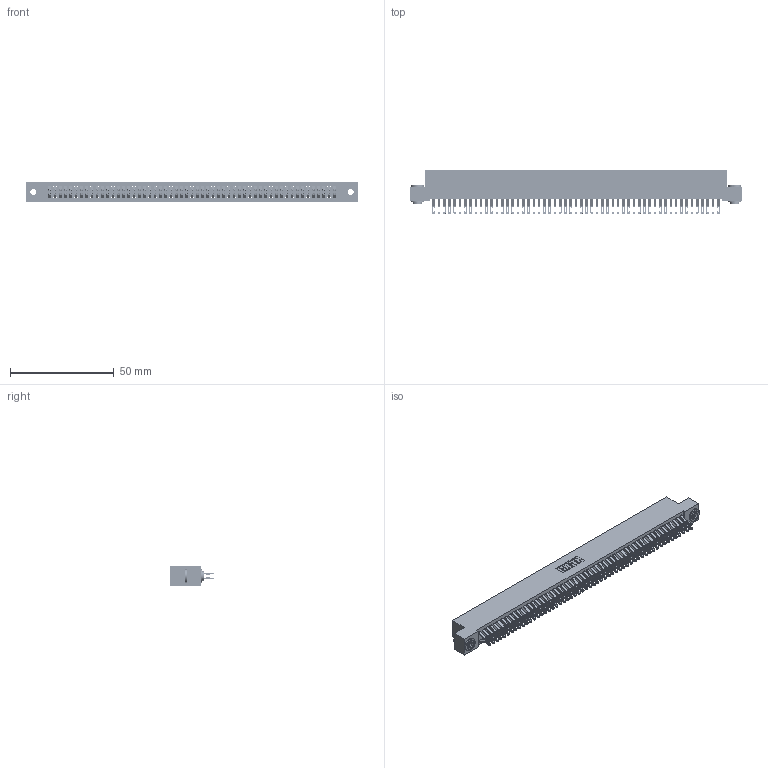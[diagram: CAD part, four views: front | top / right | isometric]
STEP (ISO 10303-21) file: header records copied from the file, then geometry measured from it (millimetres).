
FILE_DESCRIPTION (( 'STEP AP203' ), '1' );
FILE_NAME ('342-110-555-203.STEP', '2018-08-14T11:41:17', ( '' ), ( '' ), 'SwSTEP 2.0', 'SolidWorks 2016', '' );
FILE_SCHEMA (( 'CONFIG_CONTROL_DESIGN' ));
Length unit declared in the file: inch
Products named in the file (4): 342-110-555-203; 342 Part_.156 TH; 345-292-001_555 Tail; 342-250-002_345-250-002-102
Assembly tree (113 placements, depth 2):
  342-110-555-203
    342 Part_.156 TH
    345-292-001_555 Tail  x110
    342-250-002_345-250-002-102  x2
Bounding box: 160.02 x 21.47 x 9.4 mm (x, y, z)
Volume: 14767.8 mm3; surface area: 25637 mm2
Topology: 113 solids, 113 shells, 6528 faces, 20505 edges, 13666 vertices
Faces by surface type: plane 3816, cylinder 2704, cone 8
Entity records: 34546 total; most frequent: CARTESIAN_POINT 5719, ORIENTED_EDGE 5618, DIRECTION 4867, EDGE_CURVE 2809, VECTOR 2637, LINE 2637, VERTEX_POINT 1870, AXIS2_PLACEMENT_3D 1115
